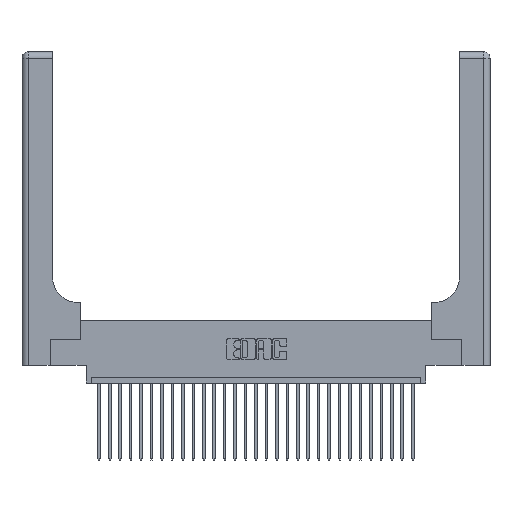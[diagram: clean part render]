
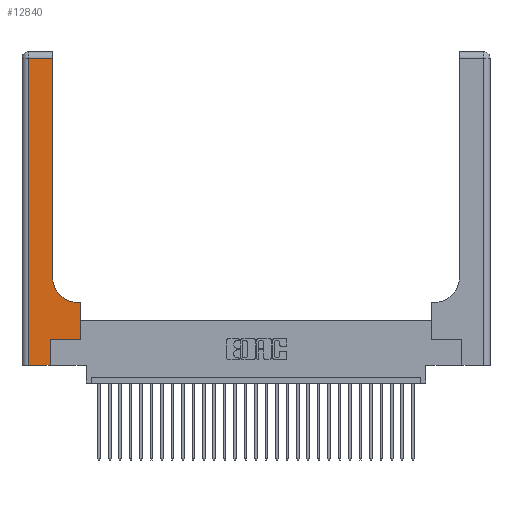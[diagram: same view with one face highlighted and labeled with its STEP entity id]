
A CAD part, top view. The second image highlights one B-rep face of the part: STEP entity #12840.
In plain terms, the highlighted planar face has unit normal (0, 0, 1).
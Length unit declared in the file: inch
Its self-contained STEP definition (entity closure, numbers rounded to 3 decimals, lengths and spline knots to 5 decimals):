
#40 = EDGE_CURVE ( 'NONE', #14745, #27351, #14355, .T. ) ;
#551 = LINE ( 'NONE', #17769, #22868 ) ;
#1575 = CARTESIAN_POINT ( 'NONE',  ( 0., 3., 0.37 ) ) ;
#1678 = DIRECTION ( 'NONE',  ( 0., 0., -1. ) ) ;
#2053 = FACE_OUTER_BOUND ( 'NONE', #12487, .T. ) ;
#2923 = VERTEX_POINT ( 'NONE', #29790 ) ;
#2925 = LINE ( 'NONE', #18932, #26249 ) ;
#3031 = CARTESIAN_POINT ( 'NONE',  ( 0.5415, 0.85, 0.37 ) ) ;
#3291 = ORIENTED_EDGE ( 'NONE', *, *, #6991, .T. ) ;
#3907 = EDGE_CURVE ( 'NONE', #6329, #2923, #27806, .T. ) ;
#4178 = LINE ( 'NONE', #22306, #21741 ) ;
#4217 = ORIENTED_EDGE ( 'NONE', *, *, #27062, .T. ) ;
#4483 = VECTOR ( 'NONE', #18007, 39.37008 ) ;
#5886 = DIRECTION ( 'NONE',  ( -1., 0., 0. ) ) ;
#6069 = DIRECTION ( 'NONE',  ( 1., 0., 0. ) ) ;
#6329 = VERTEX_POINT ( 'NONE', #8455 ) ;
#6545 = AXIS2_PLACEMENT_3D ( 'NONE', #1575, #1678, #22587 ) ;
#6572 = VERTEX_POINT ( 'NONE', #23945 ) ;
#6991 = EDGE_CURVE ( 'NONE', #6572, #14745, #4178, .T. ) ;
#7121 = EDGE_CURVE ( 'NONE', #16556, #12833, #10736, .T. ) ;
#7782 = VERTEX_POINT ( 'NONE', #28764 ) ;
#7789 = DIRECTION ( 'NONE',  ( 1., 0., 0. ) ) ;
#8115 = ORIENTED_EDGE ( 'NONE', *, *, #7121, .T. ) ;
#8455 = CARTESIAN_POINT ( 'NONE',  ( 0.06, 2.94, 0.37 ) ) ;
#8516 = LINE ( 'NONE', #10016, #24601 ) ;
#8638 = VECTOR ( 'NONE', #5886, 39.37008 ) ;
#8996 = ORIENTED_EDGE ( 'NONE', *, *, #9562, .T. ) ;
#9562 = EDGE_CURVE ( 'NONE', #7782, #6329, #10172, .T. ) ;
#9918 = EDGE_CURVE ( 'NONE', #12833, #7782, #2925, .T. ) ;
#10016 = CARTESIAN_POINT ( 'NONE',  ( 0.5585, 0.25, 0.37 ) ) ;
#10172 = LINE ( 'NONE', #11943, #24112 ) ;
#10185 = ORIENTED_EDGE ( 'NONE', *, *, #12506, .T. ) ;
#10411 = DIRECTION ( 'NONE',  ( -1., 0., 0. ) ) ;
#10437 = ORIENTED_EDGE ( 'NONE', *, *, #40, .T. ) ;
#10736 = CIRCLE ( 'NONE', #17736, 0.25 ) ;
#11943 = CARTESIAN_POINT ( 'NONE',  ( 0., 2.94, 0.37 ) ) ;
#12487 = EDGE_LOOP ( 'NONE', ( #25554, #8996, #24927, #10185, #3291, #10437, #4217, #15147, #8115 ) ) ;
#12506 = EDGE_CURVE ( 'NONE', #2923, #6572, #551, .T. ) ;
#12617 = PLANE ( 'NONE',  #6545 ) ;
#12833 = VERTEX_POINT ( 'NONE', #29029 ) ;
#12840 = ADVANCED_FACE ( 'NONE', ( #2053 ), #12617, .F. ) ;
#12949 = DIRECTION ( 'NONE',  ( 0., 1., 0. ) ) ;
#14355 = LINE ( 'NONE', #25439, #18760 ) ;
#14627 = DIRECTION ( 'NONE',  ( 0., 1., 0. ) ) ;
#14745 = VERTEX_POINT ( 'NONE', #26051 ) ;
#14911 = EDGE_CURVE ( 'NONE', #29633, #16556, #19215, .T. ) ;
#15147 = ORIENTED_EDGE ( 'NONE', *, *, #14911, .T. ) ;
#16556 = VERTEX_POINT ( 'NONE', #21389 ) ;
#17736 = AXIS2_PLACEMENT_3D ( 'NONE', #3031, #28745, #7789 ) ;
#17769 = CARTESIAN_POINT ( 'NONE',  ( 0., 0., 0.37 ) ) ;
#18007 = DIRECTION ( 'NONE',  ( 0., -1., 0. ) ) ;
#18029 = CARTESIAN_POINT ( 'NONE',  ( 0.5585, 0.6, 0.37 ) ) ;
#18760 = VECTOR ( 'NONE', #25241, 39.37008 ) ;
#18932 = CARTESIAN_POINT ( 'NONE',  ( 0.2915, 3., 0.37 ) ) ;
#19215 = LINE ( 'NONE', #29047, #8638 ) ;
#21389 = CARTESIAN_POINT ( 'NONE',  ( 0.5415, 0.6, 0.37 ) ) ;
#21741 = VECTOR ( 'NONE', #12949, 39.37008 ) ;
#22306 = CARTESIAN_POINT ( 'NONE',  ( 0.269, 0., 0.37 ) ) ;
#22587 = DIRECTION ( 'NONE',  ( -1., 0., 0. ) ) ;
#22868 = VECTOR ( 'NONE', #6069, 39.37008 ) ;
#23273 = CARTESIAN_POINT ( 'NONE',  ( 0.5585, 0.25, 0.37 ) ) ;
#23945 = CARTESIAN_POINT ( 'NONE',  ( 0.269, 0., 0.37 ) ) ;
#24112 = VECTOR ( 'NONE', #10411, 39.37008 ) ;
#24601 = VECTOR ( 'NONE', #28655, 39.37008 ) ;
#24927 = ORIENTED_EDGE ( 'NONE', *, *, #3907, .T. ) ;
#25241 = DIRECTION ( 'NONE',  ( 1., 0., 0. ) ) ;
#25439 = CARTESIAN_POINT ( 'NONE',  ( 0.269, 0.25, 0.37 ) ) ;
#25554 = ORIENTED_EDGE ( 'NONE', *, *, #9918, .T. ) ;
#26051 = CARTESIAN_POINT ( 'NONE',  ( 0.269, 0.25, 0.37 ) ) ;
#26249 = VECTOR ( 'NONE', #14627, 39.37008 ) ;
#27062 = EDGE_CURVE ( 'NONE', #27351, #29633, #8516, .T. ) ;
#27351 = VERTEX_POINT ( 'NONE', #23273 ) ;
#27806 = LINE ( 'NONE', #28476, #4483 ) ;
#28476 = CARTESIAN_POINT ( 'NONE',  ( 0.06, 3., 0.37 ) ) ;
#28655 = DIRECTION ( 'NONE',  ( 0., 1., 0. ) ) ;
#28745 = DIRECTION ( 'NONE',  ( 0., 0., -1. ) ) ;
#28764 = CARTESIAN_POINT ( 'NONE',  ( 0.2915, 2.94, 0.37 ) ) ;
#29029 = CARTESIAN_POINT ( 'NONE',  ( 0.2915, 0.85, 0.37 ) ) ;
#29047 = CARTESIAN_POINT ( 'NONE',  ( 0.2915, 0.6, 0.37 ) ) ;
#29633 = VERTEX_POINT ( 'NONE', #18029 ) ;
#29790 = CARTESIAN_POINT ( 'NONE',  ( 0.06, 0., 0.37 ) ) ;
